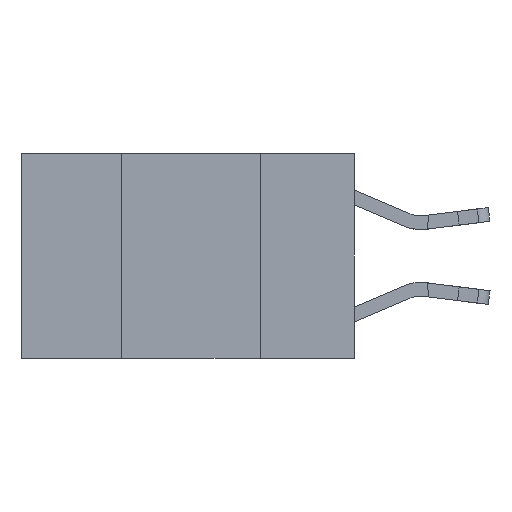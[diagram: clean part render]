
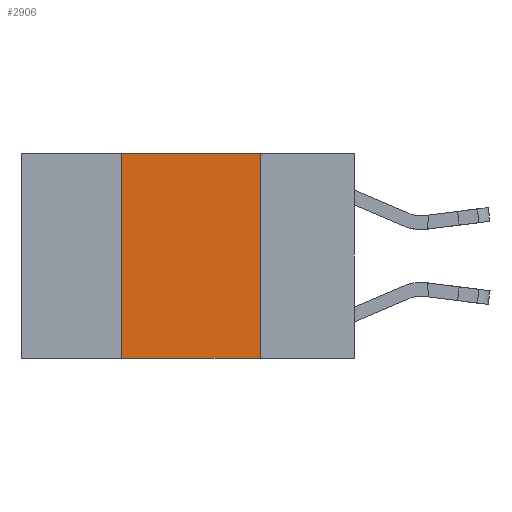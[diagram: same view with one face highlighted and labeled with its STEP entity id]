
A CAD part, left-side view. The second image highlights one B-rep face of the part: STEP entity #2906.
In plain terms, the highlighted planar face has unit normal (-1, 0, 0).
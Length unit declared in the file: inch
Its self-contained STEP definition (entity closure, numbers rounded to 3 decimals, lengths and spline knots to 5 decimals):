
#386 = VECTOR ( 'NONE', #12802, 39.37008 ) ;
#449 = VERTEX_POINT ( 'NONE', #7262 ) ;
#768 = CARTESIAN_POINT ( 'NONE',  ( 0., 0.42, 0. ) ) ;
#1181 = ORIENTED_EDGE ( 'NONE', *, *, #18177, .F. ) ;
#1739 = DIRECTION ( 'NONE',  ( 0., -1., 0. ) ) ;
#2245 = DIRECTION ( 'NONE',  ( 0., 0., 1. ) ) ;
#2906 = ADVANCED_FACE ( 'NONE', ( #19982 ), #17828, .F. ) ;
#3219 = CARTESIAN_POINT ( 'NONE',  ( 0., 0.17, 0. ) ) ;
#3357 = CARTESIAN_POINT ( 'NONE',  ( 0., 0.6, 0. ) ) ;
#3591 = VECTOR ( 'NONE', #9566, 39.37008 ) ;
#4038 = AXIS2_PLACEMENT_3D ( 'NONE', #11643, #5365, #16371 ) ;
#4142 = VECTOR ( 'NONE', #2245, 39.37008 ) ;
#4555 = VERTEX_POINT ( 'NONE', #17420 ) ;
#4624 = LINE ( 'NONE', #11682, #4142 ) ;
#5299 = EDGE_CURVE ( 'NONE', #11193, #9457, #20239, .T. ) ;
#5321 = VECTOR ( 'NONE', #1739, 39.37008 ) ;
#5365 = DIRECTION ( 'NONE',  ( 1., 0., 0. ) ) ;
#5841 = ORIENTED_EDGE ( 'NONE', *, *, #19210, .T. ) ;
#7262 = CARTESIAN_POINT ( 'NONE',  ( 0., 0.17, -0.37 ) ) ;
#9457 = VERTEX_POINT ( 'NONE', #14064 ) ;
#9566 = DIRECTION ( 'NONE',  ( 0., 0., -1. ) ) ;
#11180 = CARTESIAN_POINT ( 'NONE',  ( 0., 0.6, -0.37 ) ) ;
#11193 = VERTEX_POINT ( 'NONE', #768 ) ;
#11643 = CARTESIAN_POINT ( 'NONE',  ( 0., 0.6, 0. ) ) ;
#11682 = CARTESIAN_POINT ( 'NONE',  ( 0., 0.42, 0. ) ) ;
#12759 = ORIENTED_EDGE ( 'NONE', *, *, #16114, .F. ) ;
#12794 = EDGE_LOOP ( 'NONE', ( #12759, #17357, #1181, #5841 ) ) ;
#12802 = DIRECTION ( 'NONE',  ( 0., -1., 0. ) ) ;
#14064 = CARTESIAN_POINT ( 'NONE',  ( 0., 0.17, 0. ) ) ;
#16114 = EDGE_CURVE ( 'NONE', #9457, #449, #16645, .T. ) ;
#16371 = DIRECTION ( 'NONE',  ( 0., 0., -1. ) ) ;
#16645 = LINE ( 'NONE', #3219, #3591 ) ;
#17357 = ORIENTED_EDGE ( 'NONE', *, *, #5299, .F. ) ;
#17420 = CARTESIAN_POINT ( 'NONE',  ( 0., 0.42, -0.37 ) ) ;
#17828 = PLANE ( 'NONE',  #4038 ) ;
#18177 = EDGE_CURVE ( 'NONE', #4555, #11193, #4624, .T. ) ;
#18323 = LINE ( 'NONE', #11180, #5321 ) ;
#19210 = EDGE_CURVE ( 'NONE', #4555, #449, #18323, .T. ) ;
#19982 = FACE_OUTER_BOUND ( 'NONE', #12794, .T. ) ;
#20239 = LINE ( 'NONE', #3357, #386 ) ;
